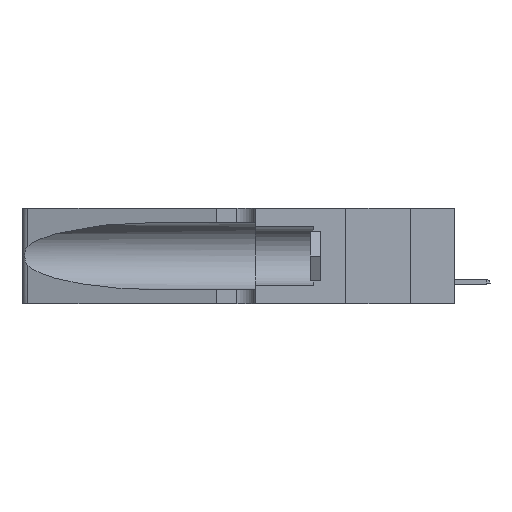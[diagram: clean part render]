
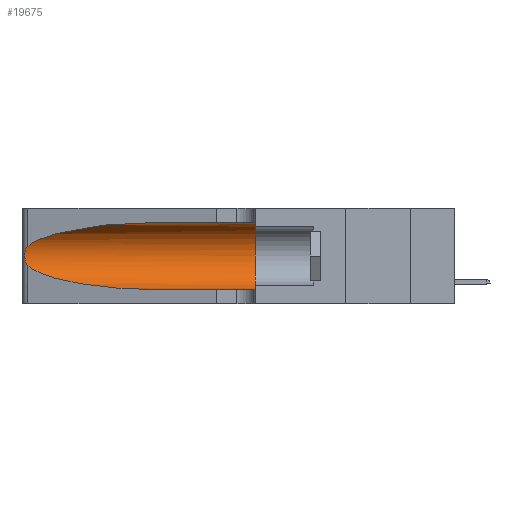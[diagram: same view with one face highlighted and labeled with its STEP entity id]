
A CAD part, left-side view. The second image highlights one B-rep face of the part: STEP entity #19675.
In plain terms, the highlighted cylindrical face has radius 3.308 mm (diameter 6.617 mm), a partial arc.
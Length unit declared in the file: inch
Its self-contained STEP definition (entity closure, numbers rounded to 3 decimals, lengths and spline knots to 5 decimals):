
#619 = VECTOR ( 'NONE', #26237, 39.37008 ) ;
#1118 = EDGE_CURVE ( 'NONE', #1632, #18533, #19808, .T. ) ;
#1632 = VERTEX_POINT ( 'NONE', #19225 ) ;
#1761 =( BOUNDED_CURVE ( )  B_SPLINE_CURVE ( 3, ( #2076, #26849, #34329, #2433 ),
 .UNSPECIFIED., .F., .F. ) 
 B_SPLINE_CURVE_WITH_KNOTS ( ( 4, 4 ),
 ( 1.5708, 2.84003 ),
 .UNSPECIFIED. ) 
 CURVE ( )  GEOMETRIC_REPRESENTATION_ITEM ( )  RATIONAL_B_SPLINE_CURVE ( ( 1., 0.87, 0.87, 1. ) ) 
 REPRESENTATION_ITEM ( '' )  );
#2001 = CARTESIAN_POINT ( 'NONE',  ( 0.1305, 0.35, 0.185 ) ) ;
#2076 = CARTESIAN_POINT ( 'NONE',  ( 0.1305, 0.72297, 0.31525 ) ) ;
#2319 = EDGE_CURVE ( 'NONE', #19570, #32900, #28918, .T. ) ;
#2350 = CARTESIAN_POINT ( 'NONE',  ( 0.25854, 1.2359, 0.20912 ) ) ;
#2433 = CARTESIAN_POINT ( 'NONE',  ( 0.25487, 1.22718, 0.22369 ) ) ;
#3170 = FACE_OUTER_BOUND ( 'NONE', #21494, .T. ) ;
#3533 = ORIENTED_EDGE ( 'NONE', *, *, #10694, .T. ) ;
#4512 = CARTESIAN_POINT ( 'NONE',  ( 0.1305, 1.61858, 0.05475 ) ) ;
#5398 = CARTESIAN_POINT ( 'NONE',  ( 0.25555, 1.22993, 0.14849 ) ) ;
#6586 = LINE ( 'NONE', #33837, #9495 ) ;
#6712 = CIRCLE ( 'NONE', #23180, 0.13025 ) ;
#6723 = VERTEX_POINT ( 'NONE', #8226 ) ;
#7926 =( BOUNDED_CURVE ( )  B_SPLINE_CURVE ( 3, ( #27909, #9388, #20423, #31294 ),
 .UNSPECIFIED., .F., .F. ) 
 B_SPLINE_CURVE_WITH_KNOTS ( ( 4, 4 ),
 ( 3.44316, 4.71239 ),
 .UNSPECIFIED. ) 
 CURVE ( )  GEOMETRIC_REPRESENTATION_ITEM ( )  RATIONAL_B_SPLINE_CURVE ( ( 1., 0.87, 0.87, 1. ) ) 
 REPRESENTATION_ITEM ( '' )  );
#8226 = CARTESIAN_POINT ( 'NONE',  ( 0.1305, 0.72297, 0.31525 ) ) ;
#8947 = EDGE_CURVE ( 'NONE', #6723, #14507, #6586, .T. ) ;
#9233 = ORIENTED_EDGE ( 'NONE', *, *, #34143, .F. ) ;
#9388 = CARTESIAN_POINT ( 'NONE',  ( 0.2373, 1.15595, 0.08982 ) ) ;
#9495 = VECTOR ( 'NONE', #20794, 39.37008 ) ;
#9705 = DIRECTION ( 'NONE',  ( 0., 1., 0. ) ) ;
#10694 = EDGE_CURVE ( 'NONE', #6723, #1632, #1761, .T. ) ;
#10742 = CARTESIAN_POINT ( 'NONE',  ( 0.25555, 1.22994, 0.2215 ) ) ;
#10917 = CARTESIAN_POINT ( 'NONE',  ( 0.25487, 1.22718, 0.22369 ) ) ;
#12354 = CARTESIAN_POINT ( 'NONE',  ( 0.1305, 0.35, 0.05475 ) ) ;
#14233 = DIRECTION ( 'NONE',  ( 0., -1., 0. ) ) ;
#14507 = VERTEX_POINT ( 'NONE', #27328 ) ;
#14730 = CARTESIAN_POINT ( 'NONE',  ( 0.1305, 0.72297, 0.05475 ) ) ;
#17500 = AXIS2_PLACEMENT_3D ( 'NONE', #22400, #14233, #19740 ) ;
#18533 = VERTEX_POINT ( 'NONE', #26262 ) ;
#19225 = CARTESIAN_POINT ( 'NONE',  ( 0.25487, 1.22718, 0.22369 ) ) ;
#19265 = CARTESIAN_POINT ( 'NONE',  ( 0.26017, 1.23833, 0.17102 ) ) ;
#19541 = EDGE_CURVE ( 'NONE', #18533, #19570, #7926, .T. ) ;
#19570 = VERTEX_POINT ( 'NONE', #14730 ) ;
#19675 = ADVANCED_FACE ( 'NONE', ( #3170 ), #27930, .F. ) ;
#19740 = DIRECTION ( 'NONE',  ( 0., 0., -1. ) ) ;
#19808 = B_SPLINE_CURVE_WITH_KNOTS ( 'NONE', 3,
 ( #10917, #10742, #24607, #21595, #2350, #27296, #32469, #24080, #19265, #30153, #34952, #21411, #5398, #32644 ),
 .UNSPECIFIED., .F., .F.,
 ( 4, 2, 2, 2, 2, 2, 4 ),
 ( 0., 0.00027, 0.00053, 0.00107, 0.0016, 0.00187, 0.00214 ),
 .UNSPECIFIED. ) ;
#20380 = DIRECTION ( 'NONE',  ( 0., 0., 1. ) ) ;
#20423 = CARTESIAN_POINT ( 'NONE',  ( 0.18966, 0.96281, 0.05475 ) ) ;
#20794 = DIRECTION ( 'NONE',  ( 0., -1., 0. ) ) ;
#21411 = CARTESIAN_POINT ( 'NONE',  ( 0.25639, 1.23186, 0.15144 ) ) ;
#21494 = EDGE_LOOP ( 'NONE', ( #3533, #23097, #22257, #23495, #9233, #28421 ) ) ;
#21595 = CARTESIAN_POINT ( 'NONE',  ( 0.25787, 1.23484, 0.2124 ) ) ;
#22257 = ORIENTED_EDGE ( 'NONE', *, *, #19541, .T. ) ;
#22400 = CARTESIAN_POINT ( 'NONE',  ( 0.1305, 1.61858, 0.185 ) ) ;
#23097 = ORIENTED_EDGE ( 'NONE', *, *, #1118, .T. ) ;
#23180 = AXIS2_PLACEMENT_3D ( 'NONE', #2001, #9705, #20380 ) ;
#23495 = ORIENTED_EDGE ( 'NONE', *, *, #2319, .T. ) ;
#24080 = CARTESIAN_POINT ( 'NONE',  ( 0.26075, 1.23896, 0.178 ) ) ;
#24607 = CARTESIAN_POINT ( 'NONE',  ( 0.25639, 1.23184, 0.21858 ) ) ;
#26237 = DIRECTION ( 'NONE',  ( 0., -1., 0. ) ) ;
#26262 = CARTESIAN_POINT ( 'NONE',  ( 0.25487, 1.22718, 0.14631 ) ) ;
#26849 = CARTESIAN_POINT ( 'NONE',  ( 0.18966, 0.96281, 0.31525 ) ) ;
#27296 = CARTESIAN_POINT ( 'NONE',  ( 0.26018, 1.23835, 0.19895 ) ) ;
#27328 = CARTESIAN_POINT ( 'NONE',  ( 0.1305, 0.35, 0.31525 ) ) ;
#27909 = CARTESIAN_POINT ( 'NONE',  ( 0.25487, 1.22718, 0.14631 ) ) ;
#27930 = CYLINDRICAL_SURFACE ( 'NONE', #17500, 0.13025 ) ;
#28421 = ORIENTED_EDGE ( 'NONE', *, *, #8947, .F. ) ;
#28918 = LINE ( 'NONE', #4512, #619 ) ;
#30153 = CARTESIAN_POINT ( 'NONE',  ( 0.25856, 1.23593, 0.16098 ) ) ;
#31294 = CARTESIAN_POINT ( 'NONE',  ( 0.1305, 0.72297, 0.05475 ) ) ;
#32469 = CARTESIAN_POINT ( 'NONE',  ( 0.26075, 1.23896, 0.19203 ) ) ;
#32644 = CARTESIAN_POINT ( 'NONE',  ( 0.25487, 1.22718, 0.14631 ) ) ;
#32900 = VERTEX_POINT ( 'NONE', #12354 ) ;
#33837 = CARTESIAN_POINT ( 'NONE',  ( 0.1305, 1.61858, 0.31525 ) ) ;
#34143 = EDGE_CURVE ( 'NONE', #14507, #32900, #6712, .T. ) ;
#34329 = CARTESIAN_POINT ( 'NONE',  ( 0.2373, 1.15595, 0.28018 ) ) ;
#34952 = CARTESIAN_POINT ( 'NONE',  ( 0.25789, 1.23486, 0.15765 ) ) ;
